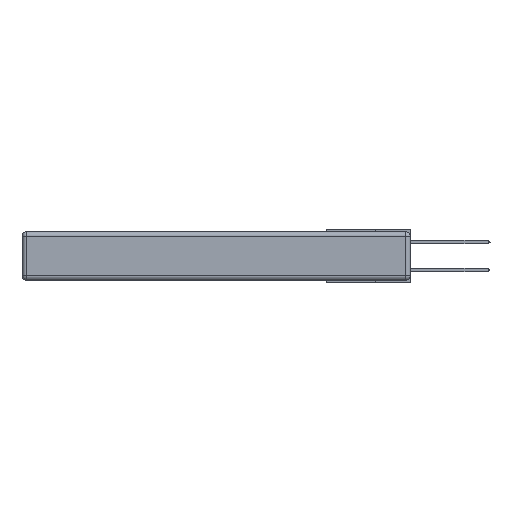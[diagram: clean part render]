
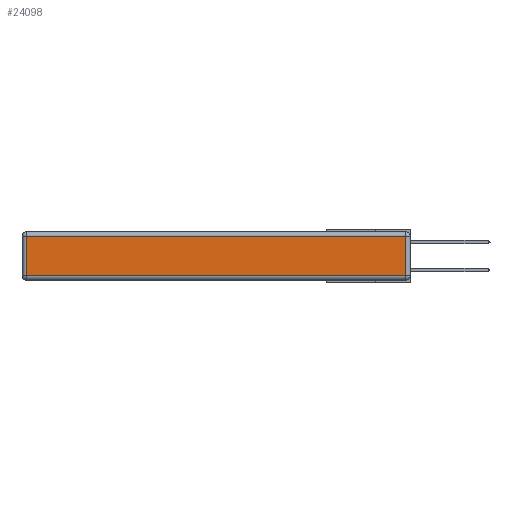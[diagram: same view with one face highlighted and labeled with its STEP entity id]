
A CAD part, left-side view. The second image highlights one B-rep face of the part: STEP entity #24098.
In plain terms, the highlighted planar face has unit normal (-1, 0, 0).
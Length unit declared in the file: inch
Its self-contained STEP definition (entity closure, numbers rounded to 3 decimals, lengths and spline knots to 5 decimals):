
#45 = LINE ( 'NONE', #9291, #1611 ) ;
#622 = EDGE_CURVE ( 'NONE', #7931, #7825, #16493, .T. ) ;
#1611 = VECTOR ( 'NONE', #7515, 39.37008 ) ;
#2215 = CARTESIAN_POINT ( 'NONE',  ( 0., 2.72, -0.313 ) ) ;
#2551 = VERTEX_POINT ( 'NONE', #2215 ) ;
#3141 = CARTESIAN_POINT ( 'NONE',  ( 0., 0., -0.343 ) ) ;
#4062 = DIRECTION ( 'NONE',  ( 0., 1., 0. ) ) ;
#4151 = CARTESIAN_POINT ( 'NONE',  ( 0., 2.75, -0.03 ) ) ;
#4405 = VECTOR ( 'NONE', #5231, 39.37008 ) ;
#4591 = AXIS2_PLACEMENT_3D ( 'NONE', #3141, #7359, #6992 ) ;
#4663 = CARTESIAN_POINT ( 'NONE',  ( 0., 0.03, -0.313 ) ) ;
#5231 = DIRECTION ( 'NONE',  ( 0., 0., -1. ) ) ;
#6328 = ORIENTED_EDGE ( 'NONE', *, *, #18083, .T. ) ;
#6992 = DIRECTION ( 'NONE',  ( 0., 0., 1. ) ) ;
#7233 = CARTESIAN_POINT ( 'NONE',  ( 0., 0.03, -0.343 ) ) ;
#7359 = DIRECTION ( 'NONE',  ( -1., 0., 0. ) ) ;
#7515 = DIRECTION ( 'NONE',  ( 0., -1., 0. ) ) ;
#7825 = VERTEX_POINT ( 'NONE', #18348 ) ;
#7931 = VERTEX_POINT ( 'NONE', #4663 ) ;
#9098 = VECTOR ( 'NONE', #20900, 39.37008 ) ;
#9291 = CARTESIAN_POINT ( 'NONE',  ( 0., 0., -0.313 ) ) ;
#9694 = LINE ( 'NONE', #18551, #4405 ) ;
#9862 = EDGE_CURVE ( 'NONE', #15861, #2551, #9694, .T. ) ;
#10836 = ORIENTED_EDGE ( 'NONE', *, *, #622, .T. ) ;
#11877 = FACE_OUTER_BOUND ( 'NONE', #18147, .T. ) ;
#13471 = EDGE_CURVE ( 'NONE', #2551, #7931, #45, .T. ) ;
#15194 = CARTESIAN_POINT ( 'NONE',  ( 0., 2.72, -0.03 ) ) ;
#15861 = VERTEX_POINT ( 'NONE', #15194 ) ;
#16493 = LINE ( 'NONE', #7233, #9098 ) ;
#17659 = ORIENTED_EDGE ( 'NONE', *, *, #9862, .T. ) ;
#18083 = EDGE_CURVE ( 'NONE', #7825, #15861, #22443, .T. ) ;
#18147 = EDGE_LOOP ( 'NONE', ( #23335, #10836, #6328, #17659 ) ) ;
#18348 = CARTESIAN_POINT ( 'NONE',  ( 0., 0.03, -0.03 ) ) ;
#18389 = VECTOR ( 'NONE', #4062, 39.37008 ) ;
#18551 = CARTESIAN_POINT ( 'NONE',  ( 0., 2.72, -0.343 ) ) ;
#20900 = DIRECTION ( 'NONE',  ( 0., 0., 1. ) ) ;
#22443 = LINE ( 'NONE', #4151, #18389 ) ;
#23335 = ORIENTED_EDGE ( 'NONE', *, *, #13471, .T. ) ;
#24098 = ADVANCED_FACE ( 'NONE', ( #11877 ), #24808, .T. ) ;
#24808 = PLANE ( 'NONE',  #4591 ) ;
